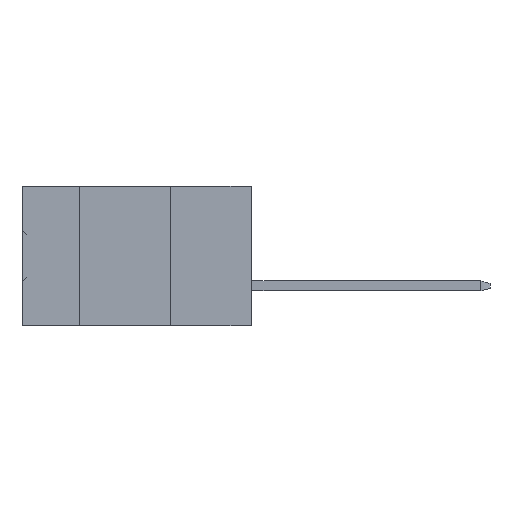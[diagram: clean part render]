
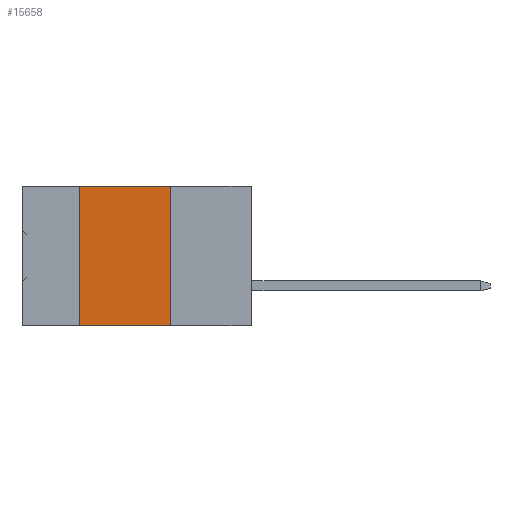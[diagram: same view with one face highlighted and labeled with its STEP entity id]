
A CAD part, left-side view. The second image highlights one B-rep face of the part: STEP entity #15658.
In plain terms, the highlighted planar face has unit normal (-1, 0, 0).
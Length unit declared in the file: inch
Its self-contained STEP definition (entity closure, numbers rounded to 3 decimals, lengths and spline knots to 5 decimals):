
#125 = CARTESIAN_POINT ( 'NONE',  ( 0., 0.72, 0. ) ) ;
#398 = CARTESIAN_POINT ( 'NONE',  ( 0., 0.254, -0.437 ) ) ;
#1767 = ORIENTED_EDGE ( 'NONE', *, *, #21838, .F. ) ;
#1906 = VECTOR ( 'NONE', #12302, 39.37008 ) ;
#2071 = LINE ( 'NONE', #25949, #30975 ) ;
#2346 = LINE ( 'NONE', #27024, #1906 ) ;
#4180 = DIRECTION ( 'NONE',  ( 0., -1., 0. ) ) ;
#4892 = VERTEX_POINT ( 'NONE', #31509 ) ;
#6249 = VECTOR ( 'NONE', #31529, 39.37008 ) ;
#7099 = DIRECTION ( 'NONE',  ( 0., 0., -1. ) ) ;
#8884 = EDGE_CURVE ( 'NONE', #15786, #27026, #26725, .T. ) ;
#10185 = CARTESIAN_POINT ( 'NONE',  ( 0., 0.254, 0. ) ) ;
#11251 = EDGE_CURVE ( 'NONE', #27026, #4892, #12894, .T. ) ;
#12302 = DIRECTION ( 'NONE',  ( 0., 0., 1. ) ) ;
#12894 = LINE ( 'NONE', #398, #15694 ) ;
#14311 = PLANE ( 'NONE',  #19938 ) ;
#15658 = ADVANCED_FACE ( 'NONE', ( #16552 ), #14311, .F. ) ;
#15694 = VECTOR ( 'NONE', #24908, 39.37008 ) ;
#15786 = VERTEX_POINT ( 'NONE', #17333 ) ;
#16552 = FACE_OUTER_BOUND ( 'NONE', #28403, .T. ) ;
#17333 = CARTESIAN_POINT ( 'NONE',  ( 0., 0.54, 0. ) ) ;
#19938 = AXIS2_PLACEMENT_3D ( 'NONE', #29512, #24380, #7099 ) ;
#20077 = EDGE_CURVE ( 'NONE', #23412, #4892, #2071, .T. ) ;
#20517 = ORIENTED_EDGE ( 'NONE', *, *, #11251, .F. ) ;
#21838 = EDGE_CURVE ( 'NONE', #23412, #15786, #2346, .T. ) ;
#22119 = ORIENTED_EDGE ( 'NONE', *, *, #20077, .T. ) ;
#23412 = VERTEX_POINT ( 'NONE', #23697 ) ;
#23697 = CARTESIAN_POINT ( 'NONE',  ( 0., 0.54, -0.437 ) ) ;
#24009 = ORIENTED_EDGE ( 'NONE', *, *, #8884, .F. ) ;
#24380 = DIRECTION ( 'NONE',  ( 1., 0., 0. ) ) ;
#24908 = DIRECTION ( 'NONE',  ( 0., 0., -1. ) ) ;
#25949 = CARTESIAN_POINT ( 'NONE',  ( 0., 0.72, -0.437 ) ) ;
#26725 = LINE ( 'NONE', #125, #6249 ) ;
#27024 = CARTESIAN_POINT ( 'NONE',  ( 0., 0.54, -0.437 ) ) ;
#27026 = VERTEX_POINT ( 'NONE', #10185 ) ;
#28403 = EDGE_LOOP ( 'NONE', ( #20517, #24009, #1767, #22119 ) ) ;
#29512 = CARTESIAN_POINT ( 'NONE',  ( 0., 0.72, 0. ) ) ;
#30975 = VECTOR ( 'NONE', #4180, 39.37008 ) ;
#31509 = CARTESIAN_POINT ( 'NONE',  ( 0., 0.254, -0.437 ) ) ;
#31529 = DIRECTION ( 'NONE',  ( 0., -1., 0. ) ) ;
